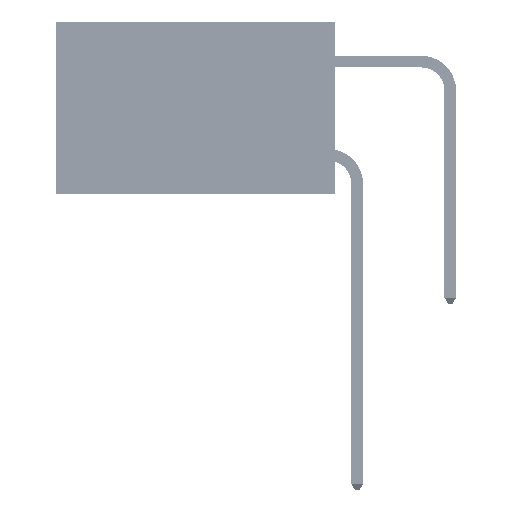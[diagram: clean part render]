
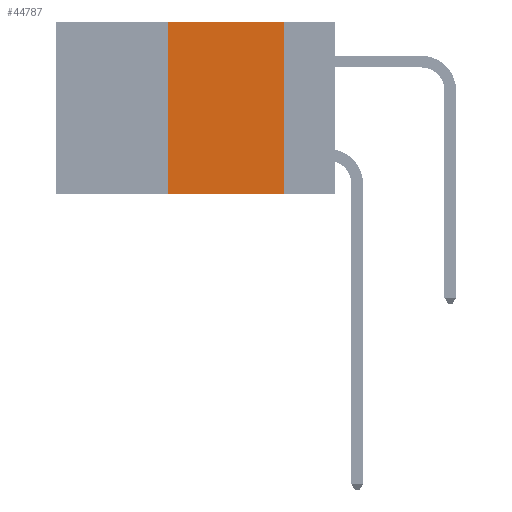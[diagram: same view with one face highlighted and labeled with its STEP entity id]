
A CAD part, left-side view. The second image highlights one B-rep face of the part: STEP entity #44787.
In plain terms, the highlighted planar face has unit normal (-1, 0, 0).
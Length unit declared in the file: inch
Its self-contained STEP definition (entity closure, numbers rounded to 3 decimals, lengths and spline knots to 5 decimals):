
#1123 = EDGE_CURVE ( 'NONE', #11891, #16946, #33279, .T. ) ;
#2311 = AXIS2_PLACEMENT_3D ( 'NONE', #11688, #53023, #28269 ) ;
#2674 = LINE ( 'NONE', #45938, #34363 ) ;
#2679 = CARTESIAN_POINT ( 'NONE',  ( 0., 0.11, 0. ) ) ;
#5077 = ORIENTED_EDGE ( 'NONE', *, *, #1123, .F. ) ;
#6848 = DIRECTION ( 'NONE',  ( 0., 0., -1. ) ) ;
#7757 = ORIENTED_EDGE ( 'NONE', *, *, #23322, .F. ) ;
#11688 = CARTESIAN_POINT ( 'NONE',  ( 0., 0.6, 0. ) ) ;
#11891 = VERTEX_POINT ( 'NONE', #43224 ) ;
#12321 = CARTESIAN_POINT ( 'NONE',  ( 0., 0.36, 0. ) ) ;
#13087 = LINE ( 'NONE', #2679, #33742 ) ;
#14839 = VECTOR ( 'NONE', #20106, 39.37008 ) ;
#15307 = EDGE_CURVE ( 'NONE', #16946, #24276, #2674, .T. ) ;
#15949 = CARTESIAN_POINT ( 'NONE',  ( 0., 0.6, -0.37 ) ) ;
#16946 = VERTEX_POINT ( 'NONE', #48145 ) ;
#18949 = EDGE_LOOP ( 'NONE', ( #7757, #35274, #5077, #30496 ) ) ;
#19265 = VERTEX_POINT ( 'NONE', #21929 ) ;
#20106 = DIRECTION ( 'NONE',  ( 0., -1., 0. ) ) ;
#21035 = VECTOR ( 'NONE', #24791, 39.37008 ) ;
#21929 = CARTESIAN_POINT ( 'NONE',  ( 0., 0.11, -0.37 ) ) ;
#22520 = CARTESIAN_POINT ( 'NONE',  ( 0., 0.11, 0. ) ) ;
#23322 = EDGE_CURVE ( 'NONE', #24276, #19265, #13087, .T. ) ;
#24276 = VERTEX_POINT ( 'NONE', #22520 ) ;
#24791 = DIRECTION ( 'NONE',  ( 0., 0., 1. ) ) ;
#26552 = FACE_OUTER_BOUND ( 'NONE', #18949, .T. ) ;
#28269 = DIRECTION ( 'NONE',  ( 0., 0., -1. ) ) ;
#30496 = ORIENTED_EDGE ( 'NONE', *, *, #32654, .T. ) ;
#32654 = EDGE_CURVE ( 'NONE', #11891, #19265, #47800, .T. ) ;
#33279 = LINE ( 'NONE', #12321, #21035 ) ;
#33742 = VECTOR ( 'NONE', #6848, 39.37008 ) ;
#34363 = VECTOR ( 'NONE', #37609, 39.37008 ) ;
#35274 = ORIENTED_EDGE ( 'NONE', *, *, #15307, .F. ) ;
#37609 = DIRECTION ( 'NONE',  ( 0., -1., 0. ) ) ;
#43224 = CARTESIAN_POINT ( 'NONE',  ( 0., 0.36, -0.37 ) ) ;
#44787 = ADVANCED_FACE ( 'NONE', ( #26552 ), #48907, .F. ) ;
#45938 = CARTESIAN_POINT ( 'NONE',  ( 0., 0.6, 0. ) ) ;
#47800 = LINE ( 'NONE', #15949, #14839 ) ;
#48145 = CARTESIAN_POINT ( 'NONE',  ( 0., 0.36, 0. ) ) ;
#48907 = PLANE ( 'NONE',  #2311 ) ;
#53023 = DIRECTION ( 'NONE',  ( 1., 0., 0. ) ) ;
